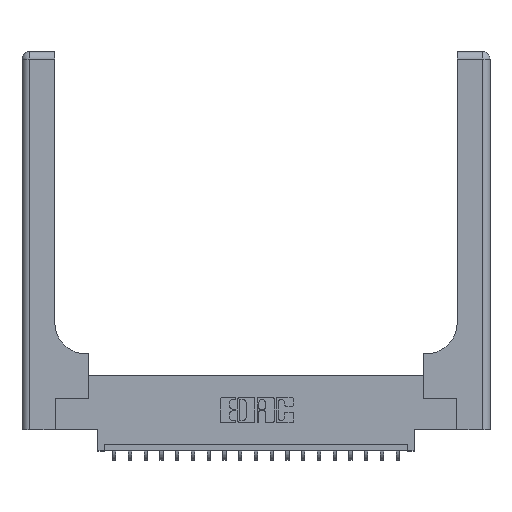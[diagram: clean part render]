
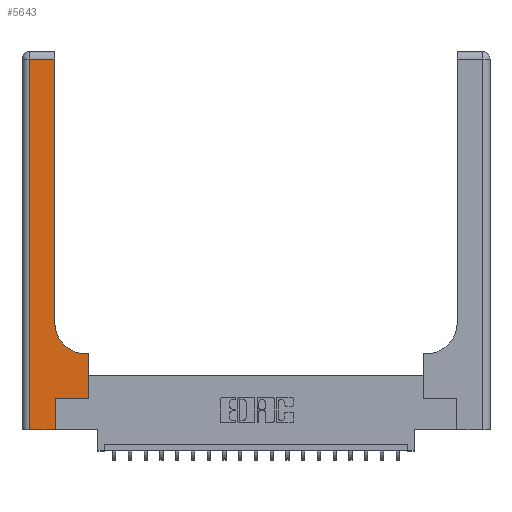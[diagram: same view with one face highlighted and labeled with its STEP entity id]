
A CAD part, top view. The second image highlights one B-rep face of the part: STEP entity #5643.
In plain terms, the highlighted planar face has unit normal (0, 0, 1).
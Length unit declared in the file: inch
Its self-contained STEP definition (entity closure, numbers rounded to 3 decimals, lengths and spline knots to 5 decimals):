
#588 = DIRECTION ( 'NONE',  ( -1., 0., 0. ) ) ;
#1076 = VERTEX_POINT ( 'NONE', #8171 ) ;
#1094 = CARTESIAN_POINT ( 'NONE',  ( 0.06, 0., 0.37 ) ) ;
#1227 = VERTEX_POINT ( 'NONE', #8638 ) ;
#1898 = AXIS2_PLACEMENT_3D ( 'NONE', #12126, #2731, #13705 ) ;
#2439 = ORIENTED_EDGE ( 'NONE', *, *, #15827, .T. ) ;
#2500 = VECTOR ( 'NONE', #8558, 39.37008 ) ;
#2731 = DIRECTION ( 'NONE',  ( 0., 0., -1. ) ) ;
#2972 = DIRECTION ( 'NONE',  ( 0., 0., -1. ) ) ;
#3030 = CARTESIAN_POINT ( 'NONE',  ( 0.528, 0.25, 0.37 ) ) ;
#3142 = VECTOR ( 'NONE', #5753, 39.37008 ) ;
#3145 = VERTEX_POINT ( 'NONE', #16511 ) ;
#3188 = CARTESIAN_POINT ( 'NONE',  ( 0.51, 0.6, 0.37 ) ) ;
#3385 = CARTESIAN_POINT ( 'NONE',  ( 0., 0., 0.37 ) ) ;
#3643 = VECTOR ( 'NONE', #13467, 39.37008 ) ;
#3657 = AXIS2_PLACEMENT_3D ( 'NONE', #12361, #2972, #13940 ) ;
#4633 = DIRECTION ( 'NONE',  ( 0., 1., 0. ) ) ;
#4657 = FACE_OUTER_BOUND ( 'NONE', #18254, .T. ) ;
#5643 = ADVANCED_FACE ( 'NONE', ( #4657 ), #7393, .F. ) ;
#5753 = DIRECTION ( 'NONE',  ( 0., 1., 0. ) ) ;
#5813 = VERTEX_POINT ( 'NONE', #6314 ) ;
#6134 = EDGE_CURVE ( 'NONE', #5813, #7247, #7792, .T. ) ;
#6161 = EDGE_CURVE ( 'NONE', #1076, #6582, #7297, .T. ) ;
#6314 = CARTESIAN_POINT ( 'NONE',  ( 0.06, 2.94, 0.37 ) ) ;
#6582 = VERTEX_POINT ( 'NONE', #14537 ) ;
#6737 = VECTOR ( 'NONE', #12207, 39.37008 ) ;
#6780 = VERTEX_POINT ( 'NONE', #7702 ) ;
#6805 = ORIENTED_EDGE ( 'NONE', *, *, #11757, .T. ) ;
#7060 = CARTESIAN_POINT ( 'NONE',  ( 0.265, 0.25, 0.37 ) ) ;
#7169 = CARTESIAN_POINT ( 'NONE',  ( 0.06, 3., 0.37 ) ) ;
#7247 = VERTEX_POINT ( 'NONE', #1094 ) ;
#7297 = LINE ( 'NONE', #10385, #3142 ) ;
#7361 = ORIENTED_EDGE ( 'NONE', *, *, #6134, .T. ) ;
#7393 = PLANE ( 'NONE',  #1898 ) ;
#7525 = LINE ( 'NONE', #3030, #19491 ) ;
#7702 = CARTESIAN_POINT ( 'NONE',  ( 0.528, 0.6, 0.37 ) ) ;
#7792 = LINE ( 'NONE', #7169, #3643 ) ;
#8009 = ORIENTED_EDGE ( 'NONE', *, *, #19043, .T. ) ;
#8171 = CARTESIAN_POINT ( 'NONE',  ( 0.26, 0.85, 0.37 ) ) ;
#8558 = DIRECTION ( 'NONE',  ( 1., 0., 0. ) ) ;
#8606 = EDGE_CURVE ( 'NONE', #13757, #1076, #11380, .T. ) ;
#8638 = CARTESIAN_POINT ( 'NONE',  ( 0.265, 0.25, 0.37 ) ) ;
#8712 = EDGE_CURVE ( 'NONE', #18162, #1227, #13087, .T. ) ;
#8926 = VECTOR ( 'NONE', #17273, 39.37008 ) ;
#9977 = CARTESIAN_POINT ( 'NONE',  ( 0., 2.94, 0.37 ) ) ;
#10308 = EDGE_CURVE ( 'NONE', #6582, #5813, #16285, .T. ) ;
#10385 = CARTESIAN_POINT ( 'NONE',  ( 0.26, 3., 0.37 ) ) ;
#10917 = ORIENTED_EDGE ( 'NONE', *, *, #8712, .T. ) ;
#11182 = DIRECTION ( 'NONE',  ( 1., 0., 0. ) ) ;
#11380 = CIRCLE ( 'NONE', #3657, 0.25 ) ;
#11757 = EDGE_CURVE ( 'NONE', #6780, #13757, #19191, .T. ) ;
#12126 = CARTESIAN_POINT ( 'NONE',  ( 0., 3., 0.37 ) ) ;
#12207 = DIRECTION ( 'NONE',  ( -1., 0., 0. ) ) ;
#12361 = CARTESIAN_POINT ( 'NONE',  ( 0.51, 0.85, 0.37 ) ) ;
#12435 = VECTOR ( 'NONE', #11182, 39.37008 ) ;
#12788 = EDGE_CURVE ( 'NONE', #1227, #3145, #18190, .T. ) ;
#12938 = LINE ( 'NONE', #3385, #12435 ) ;
#13087 = LINE ( 'NONE', #14078, #8926 ) ;
#13299 = ORIENTED_EDGE ( 'NONE', *, *, #10308, .T. ) ;
#13467 = DIRECTION ( 'NONE',  ( 0., -1., 0. ) ) ;
#13540 = ORIENTED_EDGE ( 'NONE', *, *, #6161, .T. ) ;
#13680 = CARTESIAN_POINT ( 'NONE',  ( 0.265, 0., 0.37 ) ) ;
#13705 = DIRECTION ( 'NONE',  ( -1., 0., 0. ) ) ;
#13718 = CARTESIAN_POINT ( 'NONE',  ( 0.26, 0.6, 0.37 ) ) ;
#13757 = VERTEX_POINT ( 'NONE', #3188 ) ;
#13940 = DIRECTION ( 'NONE',  ( 1., 0., 0. ) ) ;
#14078 = CARTESIAN_POINT ( 'NONE',  ( 0.265, 0., 0.37 ) ) ;
#14537 = CARTESIAN_POINT ( 'NONE',  ( 0.26, 2.94, 0.37 ) ) ;
#15827 = EDGE_CURVE ( 'NONE', #3145, #6780, #7525, .T. ) ;
#16285 = LINE ( 'NONE', #9977, #16778 ) ;
#16511 = CARTESIAN_POINT ( 'NONE',  ( 0.528, 0.25, 0.37 ) ) ;
#16594 = ORIENTED_EDGE ( 'NONE', *, *, #8606, .T. ) ;
#16778 = VECTOR ( 'NONE', #588, 39.37008 ) ;
#17273 = DIRECTION ( 'NONE',  ( 0., 1., 0. ) ) ;
#17526 = ORIENTED_EDGE ( 'NONE', *, *, #12788, .T. ) ;
#18162 = VERTEX_POINT ( 'NONE', #13680 ) ;
#18190 = LINE ( 'NONE', #7060, #2500 ) ;
#18254 = EDGE_LOOP ( 'NONE', ( #13540, #13299, #7361, #8009, #10917, #17526, #2439, #6805, #16594 ) ) ;
#19043 = EDGE_CURVE ( 'NONE', #7247, #18162, #12938, .T. ) ;
#19191 = LINE ( 'NONE', #13718, #6737 ) ;
#19491 = VECTOR ( 'NONE', #4633, 39.37008 ) ;
